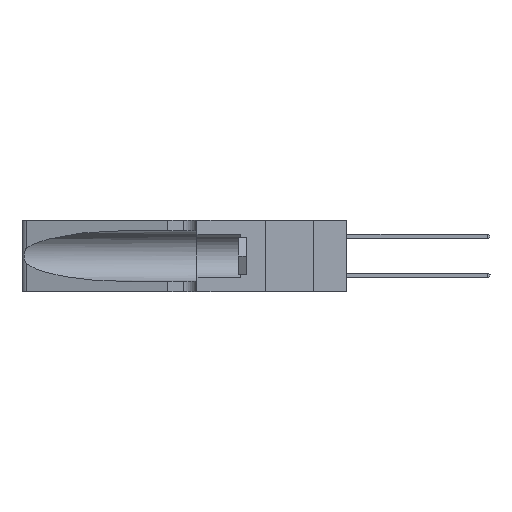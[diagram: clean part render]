
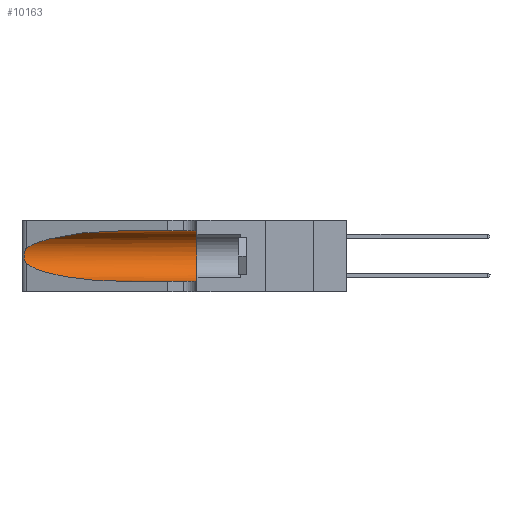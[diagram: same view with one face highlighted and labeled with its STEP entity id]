
A CAD part, left-side view. The second image highlights one B-rep face of the part: STEP entity #10163.
In plain terms, the highlighted cylindrical face has radius 3.308 mm (diameter 6.617 mm), a partial arc.
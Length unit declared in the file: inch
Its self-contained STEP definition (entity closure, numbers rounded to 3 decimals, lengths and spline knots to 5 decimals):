
#180 = DIRECTION ( 'NONE',  ( 0., 0., 1. ) ) ;
#672 = CARTESIAN_POINT ( 'NONE',  ( 0.2373, 1.15595, 0.08982 ) ) ;
#1610 = CARTESIAN_POINT ( 'NONE',  ( 0.26075, 1.23896, 0.178 ) ) ;
#1785 = EDGE_LOOP ( 'NONE', ( #19223, #23866, #25866, #27117, #5540, #6747 ) ) ;
#2744 = AXIS2_PLACEMENT_3D ( 'NONE', #26036, #13255, #180 ) ;
#3159 = VECTOR ( 'NONE', #27496, 39.37008 ) ;
#3193 = B_SPLINE_CURVE_WITH_KNOTS ( 'NONE', 3,
 ( #20909, #5989, #10306, #25233, #12453, #27359, #14598, #1610, #16715, #3862, #18876, #6079, #21000, #8254 ),
 .UNSPECIFIED., .F., .F.,
 ( 4, 2, 2, 2, 2, 2, 4 ),
 ( 0., 0.00027, 0.00053, 0.00107, 0.0016, 0.00187, 0.00214 ),
 .UNSPECIFIED. ) ;
#3862 = CARTESIAN_POINT ( 'NONE',  ( 0.25856, 1.23593, 0.16098 ) ) ;
#4401 = VERTEX_POINT ( 'NONE', #26748 ) ;
#5158 = CARTESIAN_POINT ( 'NONE',  ( 0.1305, 0.72297, 0.05475 ) ) ;
#5199 = VECTOR ( 'NONE', #26354, 39.37008 ) ;
#5205 = CARTESIAN_POINT ( 'NONE',  ( 0.1305, 0.72297, 0.05475 ) ) ;
#5540 = ORIENTED_EDGE ( 'NONE', *, *, #12161, .F. ) ;
#5860 = CIRCLE ( 'NONE', #2744, 0.13025 ) ;
#5913 = LINE ( 'NONE', #9301, #5199 ) ;
#5989 = CARTESIAN_POINT ( 'NONE',  ( 0.25555, 1.22994, 0.2215 ) ) ;
#6079 = CARTESIAN_POINT ( 'NONE',  ( 0.25639, 1.23186, 0.15144 ) ) ;
#6276 = DIRECTION ( 'NONE',  ( 0., 0., -1. ) ) ;
#6344 = FACE_OUTER_BOUND ( 'NONE', #1785, .T. ) ;
#6747 = ORIENTED_EDGE ( 'NONE', *, *, #26682, .F. ) ;
#6974 = CARTESIAN_POINT ( 'NONE',  ( 0.1305, 0.72297, 0.31525 ) ) ;
#7106 = VERTEX_POINT ( 'NONE', #24957 ) ;
#8254 = CARTESIAN_POINT ( 'NONE',  ( 0.25487, 1.22718, 0.14631 ) ) ;
#9141 = CARTESIAN_POINT ( 'NONE',  ( 0.2373, 1.15595, 0.28018 ) ) ;
#9301 = CARTESIAN_POINT ( 'NONE',  ( 0.1305, 1.61858, 0.05475 ) ) ;
#10163 = ADVANCED_FACE ( 'NONE', ( #6344 ), #10688, .F. ) ;
#10306 = CARTESIAN_POINT ( 'NONE',  ( 0.25639, 1.23184, 0.21858 ) ) ;
#10368 = VERTEX_POINT ( 'NONE', #24009 ) ;
#10688 = CYLINDRICAL_SURFACE ( 'NONE', #15608, 0.13025 ) ;
#11117 = CARTESIAN_POINT ( 'NONE',  ( 0.25487, 1.22718, 0.14631 ) ) ;
#11177 =( BOUNDED_CURVE ( )  B_SPLINE_CURVE ( 3, ( #6974, #19749, #9141, #24079 ),
 .UNSPECIFIED., .F., .T. ) 
 B_SPLINE_CURVE_WITH_KNOTS ( ( 4, 4 ),
 ( 1.5708, 2.84003 ),
 .UNSPECIFIED. ) 
 CURVE ( )  GEOMETRIC_REPRESENTATION_ITEM ( )  RATIONAL_B_SPLINE_CURVE ( ( 1., 0.87, 0.87, 1. ) ) 
 REPRESENTATION_ITEM ( '' )  );
#11557 = VERTEX_POINT ( 'NONE', #22046 ) ;
#11584 = CARTESIAN_POINT ( 'NONE',  ( 0.25487, 1.22718, 0.14631 ) ) ;
#12161 = EDGE_CURVE ( 'NONE', #10368, #7106, #5860, .T. ) ;
#12453 = CARTESIAN_POINT ( 'NONE',  ( 0.25854, 1.2359, 0.20912 ) ) ;
#13255 = DIRECTION ( 'NONE',  ( 0., 1., 0. ) ) ;
#14486 = EDGE_CURVE ( 'NONE', #4401, #24353, #3193, .T. ) ;
#14598 = CARTESIAN_POINT ( 'NONE',  ( 0.26075, 1.23896, 0.19203 ) ) ;
#14730 = CARTESIAN_POINT ( 'NONE',  ( 0.1305, 1.61858, 0.31525 ) ) ;
#14856 = EDGE_CURVE ( 'NONE', #24353, #27103, #26064, .T. ) ;
#15608 = AXIS2_PLACEMENT_3D ( 'NONE', #19076, #16896, #6276 ) ;
#16715 = CARTESIAN_POINT ( 'NONE',  ( 0.26017, 1.23833, 0.17102 ) ) ;
#16896 = DIRECTION ( 'NONE',  ( 0., -1., 0. ) ) ;
#17991 = CARTESIAN_POINT ( 'NONE',  ( 0.18966, 0.96281, 0.05475 ) ) ;
#18876 = CARTESIAN_POINT ( 'NONE',  ( 0.25789, 1.23486, 0.15765 ) ) ;
#19076 = CARTESIAN_POINT ( 'NONE',  ( 0.1305, 1.61858, 0.185 ) ) ;
#19223 = ORIENTED_EDGE ( 'NONE', *, *, #22103, .T. ) ;
#19749 = CARTESIAN_POINT ( 'NONE',  ( 0.18966, 0.96281, 0.31525 ) ) ;
#20909 = CARTESIAN_POINT ( 'NONE',  ( 0.25487, 1.22718, 0.22369 ) ) ;
#21000 = CARTESIAN_POINT ( 'NONE',  ( 0.25555, 1.22993, 0.14849 ) ) ;
#22046 = CARTESIAN_POINT ( 'NONE',  ( 0.1305, 0.72297, 0.31525 ) ) ;
#22103 = EDGE_CURVE ( 'NONE', #11557, #4401, #11177, .T. ) ;
#23866 = ORIENTED_EDGE ( 'NONE', *, *, #14486, .T. ) ;
#24009 = CARTESIAN_POINT ( 'NONE',  ( 0.1305, 0.35, 0.31525 ) ) ;
#24079 = CARTESIAN_POINT ( 'NONE',  ( 0.25487, 1.22718, 0.22369 ) ) ;
#24353 = VERTEX_POINT ( 'NONE', #11117 ) ;
#24650 = LINE ( 'NONE', #14730, #3159 ) ;
#24957 = CARTESIAN_POINT ( 'NONE',  ( 0.1305, 0.35, 0.05475 ) ) ;
#25233 = CARTESIAN_POINT ( 'NONE',  ( 0.25787, 1.23484, 0.2124 ) ) ;
#25866 = ORIENTED_EDGE ( 'NONE', *, *, #14856, .T. ) ;
#26036 = CARTESIAN_POINT ( 'NONE',  ( 0.1305, 0.35, 0.185 ) ) ;
#26064 =( BOUNDED_CURVE ( )  B_SPLINE_CURVE ( 3, ( #11584, #672, #17991, #5158 ),
 .UNSPECIFIED., .F., .F. ) 
 B_SPLINE_CURVE_WITH_KNOTS ( ( 4, 4 ),
 ( 3.44316, 4.71239 ),
 .UNSPECIFIED. ) 
 CURVE ( )  GEOMETRIC_REPRESENTATION_ITEM ( )  RATIONAL_B_SPLINE_CURVE ( ( 1., 0.87, 0.87, 1. ) ) 
 REPRESENTATION_ITEM ( '' )  );
#26354 = DIRECTION ( 'NONE',  ( 0., -1., 0. ) ) ;
#26682 = EDGE_CURVE ( 'NONE', #11557, #10368, #24650, .T. ) ;
#26748 = CARTESIAN_POINT ( 'NONE',  ( 0.25487, 1.22718, 0.22369 ) ) ;
#27017 = EDGE_CURVE ( 'NONE', #27103, #7106, #5913, .T. ) ;
#27103 = VERTEX_POINT ( 'NONE', #5205 ) ;
#27117 = ORIENTED_EDGE ( 'NONE', *, *, #27017, .T. ) ;
#27359 = CARTESIAN_POINT ( 'NONE',  ( 0.26018, 1.23835, 0.19895 ) ) ;
#27496 = DIRECTION ( 'NONE',  ( 0., -1., 0. ) ) ;
